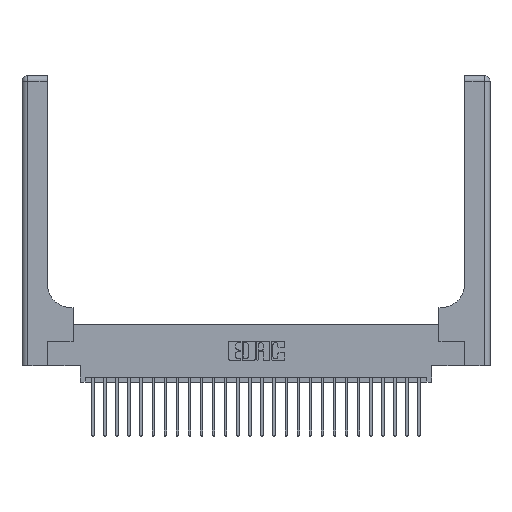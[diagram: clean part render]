
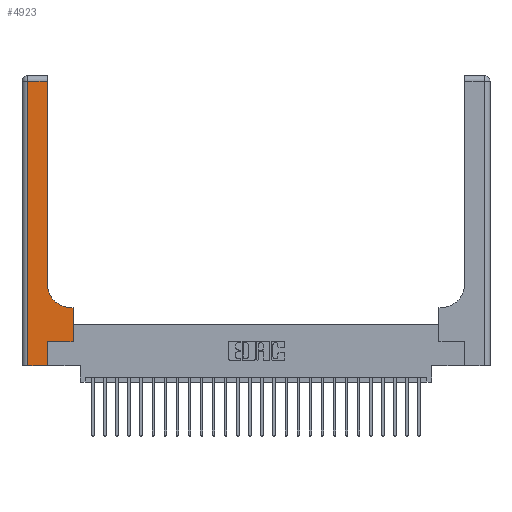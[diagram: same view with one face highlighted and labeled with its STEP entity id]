
A CAD part, top view. The second image highlights one B-rep face of the part: STEP entity #4923.
In plain terms, the highlighted planar face has unit normal (0, 0, 1).
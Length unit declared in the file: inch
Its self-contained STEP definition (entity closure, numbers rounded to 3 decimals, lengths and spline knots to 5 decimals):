
#749 = AXIS2_PLACEMENT_3D ( 'NONE', #13181, #10706, #12668 ) ;
#2689 = CARTESIAN_POINT ( 'NONE',  ( 0.265, 0., 0.37 ) ) ;
#3136 = VECTOR ( 'NONE', #20797, 39.37008 ) ;
#3297 = LINE ( 'NONE', #5512, #19928 ) ;
#3439 = CARTESIAN_POINT ( 'NONE',  ( 0.26, 0.85, 0.37 ) ) ;
#3776 = VECTOR ( 'NONE', #7454, 39.37008 ) ;
#3930 = VERTEX_POINT ( 'NONE', #25539 ) ;
#4537 = VECTOR ( 'NONE', #10687, 39.37008 ) ;
#4545 = ORIENTED_EDGE ( 'NONE', *, *, #14137, .T. ) ;
#4574 = VECTOR ( 'NONE', #13784, 39.37008 ) ;
#4752 = CARTESIAN_POINT ( 'NONE',  ( 0.06, 0., 0.37 ) ) ;
#4773 = EDGE_CURVE ( 'NONE', #15588, #23114, #24891, .T. ) ;
#4857 = VERTEX_POINT ( 'NONE', #13461 ) ;
#4923 = ADVANCED_FACE ( 'NONE', ( #23696 ), #21707, .F. ) ;
#5435 = ORIENTED_EDGE ( 'NONE', *, *, #13179, .T. ) ;
#5512 = CARTESIAN_POINT ( 'NONE',  ( 0.26, 0.6, 0.37 ) ) ;
#5706 = EDGE_CURVE ( 'NONE', #3930, #22073, #3297, .T. ) ;
#5829 = DIRECTION ( 'NONE',  ( 0., 0., -1. ) ) ;
#6382 = ORIENTED_EDGE ( 'NONE', *, *, #22212, .T. ) ;
#7454 = DIRECTION ( 'NONE',  ( 1., 0., 0. ) ) ;
#7874 = DIRECTION ( 'NONE',  ( -1., 0., 0. ) ) ;
#9138 = LINE ( 'NONE', #19248, #18566 ) ;
#9355 = AXIS2_PLACEMENT_3D ( 'NONE', #25795, #5829, #13848 ) ;
#9547 = DIRECTION ( 'NONE',  ( 0., 1., 0. ) ) ;
#10687 = DIRECTION ( 'NONE',  ( 0., 1., 0. ) ) ;
#10706 = DIRECTION ( 'NONE',  ( 0., 0., -1. ) ) ;
#10949 = CARTESIAN_POINT ( 'NONE',  ( 0.26, 3., 0.37 ) ) ;
#11030 = EDGE_LOOP ( 'NONE', ( #5435, #6382, #25241, #4545, #16638, #20254, #19229, #22621, #17254 ) ) ;
#12202 = CARTESIAN_POINT ( 'NONE',  ( 0.528, 0.25, 0.37 ) ) ;
#12649 = LINE ( 'NONE', #2689, #4537 ) ;
#12668 = DIRECTION ( 'NONE',  ( 1., 0., 0. ) ) ;
#12798 = CARTESIAN_POINT ( 'NONE',  ( 0.06, 3., 0.37 ) ) ;
#12909 = LINE ( 'NONE', #10949, #19726 ) ;
#13179 = EDGE_CURVE ( 'NONE', #23270, #14291, #12909, .T. ) ;
#13181 = CARTESIAN_POINT ( 'NONE',  ( 0.51, 0.85, 0.37 ) ) ;
#13461 = CARTESIAN_POINT ( 'NONE',  ( 0.265, 0.25, 0.37 ) ) ;
#13542 = CARTESIAN_POINT ( 'NONE',  ( 0.265, 0., 0.37 ) ) ;
#13784 = DIRECTION ( 'NONE',  ( -1., 0., 0. ) ) ;
#13848 = DIRECTION ( 'NONE',  ( -1., 0., 0. ) ) ;
#14137 = EDGE_CURVE ( 'NONE', #23114, #16788, #17691, .T. ) ;
#14291 = VERTEX_POINT ( 'NONE', #16228 ) ;
#15216 = CARTESIAN_POINT ( 'NONE',  ( 0.528, 0.25, 0.37 ) ) ;
#15588 = VERTEX_POINT ( 'NONE', #25582 ) ;
#16228 = CARTESIAN_POINT ( 'NONE',  ( 0.26, 2.94, 0.37 ) ) ;
#16638 = ORIENTED_EDGE ( 'NONE', *, *, #21590, .T. ) ;
#16788 = VERTEX_POINT ( 'NONE', #13542 ) ;
#17154 = LINE ( 'NONE', #15216, #25119 ) ;
#17254 = ORIENTED_EDGE ( 'NONE', *, *, #20615, .T. ) ;
#17691 = LINE ( 'NONE', #21613, #3776 ) ;
#17791 = EDGE_CURVE ( 'NONE', #4857, #22307, #9138, .T. ) ;
#17927 = CIRCLE ( 'NONE', #749, 0.25 ) ;
#18566 = VECTOR ( 'NONE', #21726, 39.37008 ) ;
#18959 = DIRECTION ( 'NONE',  ( 0., 1., 0. ) ) ;
#19046 = CARTESIAN_POINT ( 'NONE',  ( 0.51, 0.6, 0.37 ) ) ;
#19229 = ORIENTED_EDGE ( 'NONE', *, *, #22546, .T. ) ;
#19248 = CARTESIAN_POINT ( 'NONE',  ( 0.265, 0.25, 0.37 ) ) ;
#19562 = CARTESIAN_POINT ( 'NONE',  ( 0., 2.94, 0.37 ) ) ;
#19726 = VECTOR ( 'NONE', #18959, 39.37008 ) ;
#19928 = VECTOR ( 'NONE', #7874, 39.37008 ) ;
#20254 = ORIENTED_EDGE ( 'NONE', *, *, #17791, .T. ) ;
#20615 = EDGE_CURVE ( 'NONE', #22073, #23270, #17927, .T. ) ;
#20797 = DIRECTION ( 'NONE',  ( 0., -1., 0. ) ) ;
#21590 = EDGE_CURVE ( 'NONE', #16788, #4857, #12649, .T. ) ;
#21613 = CARTESIAN_POINT ( 'NONE',  ( 0., 0., 0.37 ) ) ;
#21707 = PLANE ( 'NONE',  #9355 ) ;
#21726 = DIRECTION ( 'NONE',  ( 1., 0., 0. ) ) ;
#22073 = VERTEX_POINT ( 'NONE', #19046 ) ;
#22212 = EDGE_CURVE ( 'NONE', #14291, #15588, #23512, .T. ) ;
#22307 = VERTEX_POINT ( 'NONE', #12202 ) ;
#22546 = EDGE_CURVE ( 'NONE', #22307, #3930, #17154, .T. ) ;
#22621 = ORIENTED_EDGE ( 'NONE', *, *, #5706, .T. ) ;
#23114 = VERTEX_POINT ( 'NONE', #4752 ) ;
#23270 = VERTEX_POINT ( 'NONE', #3439 ) ;
#23512 = LINE ( 'NONE', #19562, #4574 ) ;
#23696 = FACE_OUTER_BOUND ( 'NONE', #11030, .T. ) ;
#24891 = LINE ( 'NONE', #12798, #3136 ) ;
#25119 = VECTOR ( 'NONE', #9547, 39.37008 ) ;
#25241 = ORIENTED_EDGE ( 'NONE', *, *, #4773, .T. ) ;
#25539 = CARTESIAN_POINT ( 'NONE',  ( 0.528, 0.6, 0.37 ) ) ;
#25582 = CARTESIAN_POINT ( 'NONE',  ( 0.06, 2.94, 0.37 ) ) ;
#25795 = CARTESIAN_POINT ( 'NONE',  ( 0., 3., 0.37 ) ) ;
